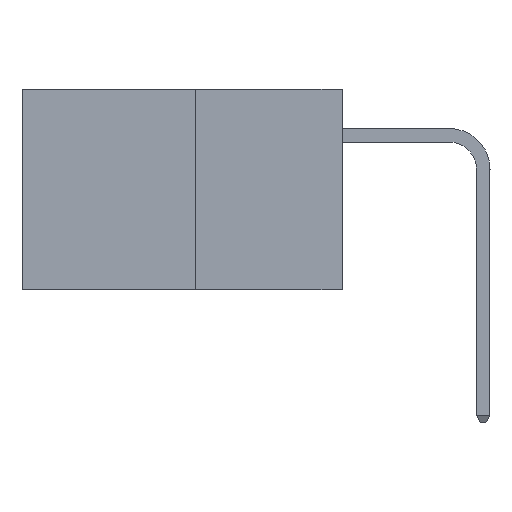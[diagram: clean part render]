
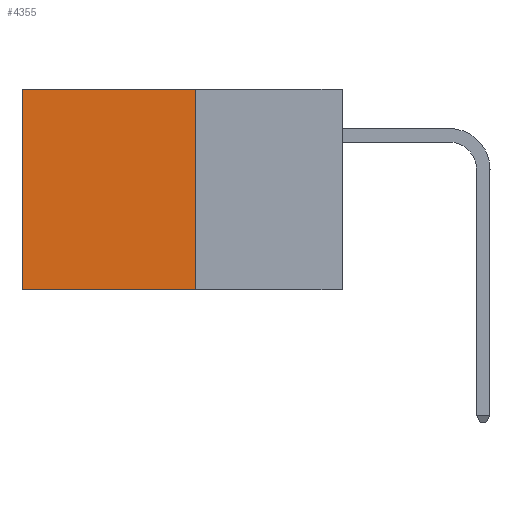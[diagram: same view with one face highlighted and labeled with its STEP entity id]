
A CAD part, left-side view. The second image highlights one B-rep face of the part: STEP entity #4355.
In plain terms, the highlighted planar face has unit normal (-1, 0, 0).
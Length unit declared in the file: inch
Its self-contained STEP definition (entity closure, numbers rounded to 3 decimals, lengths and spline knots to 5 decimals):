
#123 = CARTESIAN_POINT ( 'NONE',  ( 0.277, 0.27, -0.37 ) ) ;
#1027 = DIRECTION ( 'NONE',  ( 0., 0., -1. ) ) ;
#1049 = CARTESIAN_POINT ( 'NONE',  ( 0.277, 0.27, -0.37 ) ) ;
#1377 = VECTOR ( 'NONE', #15327, 39.37008 ) ;
#1746 = LINE ( 'NONE', #123, #10118 ) ;
#2544 = VERTEX_POINT ( 'NONE', #4985 ) ;
#3667 = VERTEX_POINT ( 'NONE', #6272 ) ;
#4074 = EDGE_CURVE ( 'NONE', #2544, #17097, #1746, .T. ) ;
#4355 = ADVANCED_FACE ( 'NONE', ( #12891 ), #9905, .F. ) ;
#4429 = LINE ( 'NONE', #17293, #13332 ) ;
#4444 = ORIENTED_EDGE ( 'NONE', *, *, #6022, .T. ) ;
#4856 = DIRECTION ( 'NONE',  ( 0., 1., 0. ) ) ;
#4985 = CARTESIAN_POINT ( 'NONE',  ( 0.277, 0.27, -0.37 ) ) ;
#5947 = EDGE_CURVE ( 'NONE', #14862, #2544, #15627, .T. ) ;
#6022 = EDGE_CURVE ( 'NONE', #14862, #3667, #4429, .T. ) ;
#6272 = CARTESIAN_POINT ( 'NONE',  ( 0.277, 0.59, 0. ) ) ;
#7931 = ORIENTED_EDGE ( 'NONE', *, *, #20933, .T. ) ;
#8239 = AXIS2_PLACEMENT_3D ( 'NONE', #20532, #11699, #1027 ) ;
#9458 = ORIENTED_EDGE ( 'NONE', *, *, #5947, .F. ) ;
#9782 = VECTOR ( 'NONE', #16244, 39.37008 ) ;
#9905 = PLANE ( 'NONE',  #8239 ) ;
#10118 = VECTOR ( 'NONE', #12647, 39.37008 ) ;
#10152 = EDGE_LOOP ( 'NONE', ( #7931, #18368, #9458, #4444 ) ) ;
#11699 = DIRECTION ( 'NONE',  ( 1., 0., 0. ) ) ;
#12647 = DIRECTION ( 'NONE',  ( 0., 1., 0. ) ) ;
#12891 = FACE_OUTER_BOUND ( 'NONE', #10152, .T. ) ;
#13332 = VECTOR ( 'NONE', #4856, 39.37008 ) ;
#14420 = CARTESIAN_POINT ( 'NONE',  ( 0.277, 0.59, -0.37 ) ) ;
#14862 = VERTEX_POINT ( 'NONE', #20914 ) ;
#15327 = DIRECTION ( 'NONE',  ( 0., 0., -1. ) ) ;
#15627 = LINE ( 'NONE', #1049, #1377 ) ;
#16244 = DIRECTION ( 'NONE',  ( 0., 0., -1. ) ) ;
#17097 = VERTEX_POINT ( 'NONE', #21433 ) ;
#17293 = CARTESIAN_POINT ( 'NONE',  ( 0.277, 0.27, 0. ) ) ;
#18368 = ORIENTED_EDGE ( 'NONE', *, *, #4074, .F. ) ;
#20532 = CARTESIAN_POINT ( 'NONE',  ( 0.277, 0.27, -0.37 ) ) ;
#20914 = CARTESIAN_POINT ( 'NONE',  ( 0.277, 0.27, 0. ) ) ;
#20933 = EDGE_CURVE ( 'NONE', #3667, #17097, #22782, .T. ) ;
#21433 = CARTESIAN_POINT ( 'NONE',  ( 0.277, 0.59, -0.37 ) ) ;
#22782 = LINE ( 'NONE', #14420, #9782 ) ;
